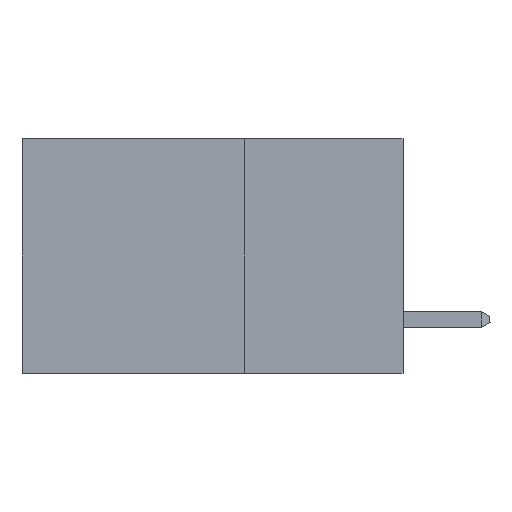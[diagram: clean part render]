
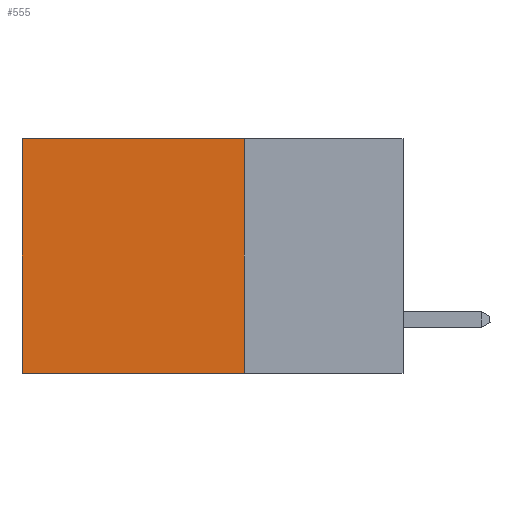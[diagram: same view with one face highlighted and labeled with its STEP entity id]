
A CAD part, left-side view. The second image highlights one B-rep face of the part: STEP entity #555.
In plain terms, the highlighted planar face has unit normal (-1, 0, 0).
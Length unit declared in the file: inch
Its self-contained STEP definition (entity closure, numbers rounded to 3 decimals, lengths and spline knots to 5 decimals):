
#64 = ORIENTED_EDGE ( 'NONE', *, *, #12807, .T. ) ;
#335 = CARTESIAN_POINT ( 'NONE',  ( 0.2875, 0.25, 0. ) ) ;
#555 = ADVANCED_FACE ( 'NONE', ( #3242 ), #12282, .F. ) ;
#1322 = EDGE_CURVE ( 'NONE', #3585, #10968, #9653, .T. ) ;
#1325 = CARTESIAN_POINT ( 'NONE',  ( 0.2875, 0.25, 0. ) ) ;
#1461 = ORIENTED_EDGE ( 'NONE', *, *, #1322, .F. ) ;
#2115 = DIRECTION ( 'NONE',  ( 0., 1., 0. ) ) ;
#3151 = VECTOR ( 'NONE', #8740, 39.37008 ) ;
#3242 = FACE_OUTER_BOUND ( 'NONE', #11533, .T. ) ;
#3585 = VERTEX_POINT ( 'NONE', #8000 ) ;
#4015 = EDGE_CURVE ( 'NONE', #3585, #12447, #6730, .T. ) ;
#4350 = DIRECTION ( 'NONE',  ( 0., 0., -1. ) ) ;
#4528 = EDGE_CURVE ( 'NONE', #10968, #6334, #11977, .T. ) ;
#4850 = VECTOR ( 'NONE', #2115, 39.37008 ) ;
#5613 = CARTESIAN_POINT ( 'NONE',  ( 0.2875, 0.6, 0. ) ) ;
#6077 = VECTOR ( 'NONE', #4350, 39.37008 ) ;
#6334 = VERTEX_POINT ( 'NONE', #8229 ) ;
#6730 = LINE ( 'NONE', #335, #3151 ) ;
#7260 = AXIS2_PLACEMENT_3D ( 'NONE', #1325, #12175, #14454 ) ;
#8000 = CARTESIAN_POINT ( 'NONE',  ( 0.2875, 0.25, 0. ) ) ;
#8229 = CARTESIAN_POINT ( 'NONE',  ( 0.2875, 0.6, -0.37 ) ) ;
#8740 = DIRECTION ( 'NONE',  ( 0., 1., 0. ) ) ;
#9653 = LINE ( 'NONE', #14137, #6077 ) ;
#9782 = LINE ( 'NONE', #5613, #12783 ) ;
#9856 = ORIENTED_EDGE ( 'NONE', *, *, #4015, .T. ) ;
#10968 = VERTEX_POINT ( 'NONE', #13295 ) ;
#11103 = CARTESIAN_POINT ( 'NONE',  ( 0.2875, 0.6, 0. ) ) ;
#11533 = EDGE_LOOP ( 'NONE', ( #64, #12920, #1461, #9856 ) ) ;
#11977 = LINE ( 'NONE', #13771, #4850 ) ;
#12175 = DIRECTION ( 'NONE',  ( 1., 0., 0. ) ) ;
#12282 = PLANE ( 'NONE',  #7260 ) ;
#12447 = VERTEX_POINT ( 'NONE', #11103 ) ;
#12783 = VECTOR ( 'NONE', #12864, 39.37008 ) ;
#12807 = EDGE_CURVE ( 'NONE', #12447, #6334, #9782, .T. ) ;
#12864 = DIRECTION ( 'NONE',  ( 0., 0., -1. ) ) ;
#12920 = ORIENTED_EDGE ( 'NONE', *, *, #4528, .F. ) ;
#13295 = CARTESIAN_POINT ( 'NONE',  ( 0.2875, 0.25, -0.37 ) ) ;
#13771 = CARTESIAN_POINT ( 'NONE',  ( 0.2875, 0.25, -0.37 ) ) ;
#14137 = CARTESIAN_POINT ( 'NONE',  ( 0.2875, 0.25, 0. ) ) ;
#14454 = DIRECTION ( 'NONE',  ( 0., 0., -1. ) ) ;
